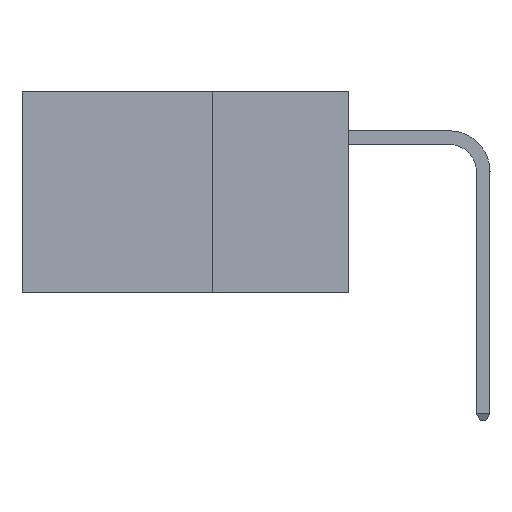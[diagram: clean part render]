
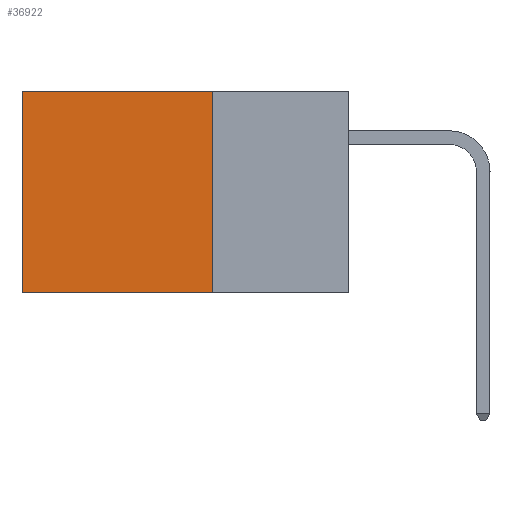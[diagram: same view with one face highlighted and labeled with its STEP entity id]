
A CAD part, left-side view. The second image highlights one B-rep face of the part: STEP entity #36922.
In plain terms, the highlighted planar face has unit normal (-1, 0, 0).
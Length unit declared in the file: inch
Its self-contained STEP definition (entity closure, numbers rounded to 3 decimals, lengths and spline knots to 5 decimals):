
#1063 = EDGE_CURVE ( 'NONE', #35926, #1633, #13323, .T. ) ;
#1204 = ORIENTED_EDGE ( 'NONE', *, *, #19303, .T. ) ;
#1633 = VERTEX_POINT ( 'NONE', #18950 ) ;
#6082 = CARTESIAN_POINT ( 'NONE',  ( 0.2875, 0.6, 0. ) ) ;
#7101 = CARTESIAN_POINT ( 'NONE',  ( 0.2875, 0.25, 0. ) ) ;
#8261 = VECTOR ( 'NONE', #16001, 39.37008 ) ;
#8582 = VECTOR ( 'NONE', #35623, 39.37008 ) ;
#9334 = VECTOR ( 'NONE', #11914, 39.37008 ) ;
#10995 = VERTEX_POINT ( 'NONE', #20126 ) ;
#11022 = EDGE_LOOP ( 'NONE', ( #1204, #17226, #28484, #34559 ) ) ;
#11562 = PLANE ( 'NONE',  #20854 ) ;
#11914 = DIRECTION ( 'NONE',  ( 0., 0., -1. ) ) ;
#13067 = CARTESIAN_POINT ( 'NONE',  ( 0.2875, 0.25, -0.37 ) ) ;
#13323 = LINE ( 'NONE', #7101, #28228 ) ;
#14456 = CARTESIAN_POINT ( 'NONE',  ( 0.2875, 0.25, 0. ) ) ;
#15670 = CARTESIAN_POINT ( 'NONE',  ( 0.2875, 0.25, 0. ) ) ;
#16001 = DIRECTION ( 'NONE',  ( 0., 1., 0. ) ) ;
#16380 = LINE ( 'NONE', #6082, #8582 ) ;
#17143 = LINE ( 'NONE', #20540, #9334 ) ;
#17226 = ORIENTED_EDGE ( 'NONE', *, *, #29145, .F. ) ;
#17474 = DIRECTION ( 'NONE',  ( 1., 0., 0. ) ) ;
#18248 = DIRECTION ( 'NONE',  ( 0., 1., 0. ) ) ;
#18950 = CARTESIAN_POINT ( 'NONE',  ( 0.2875, 0.6, 0. ) ) ;
#19303 = EDGE_CURVE ( 'NONE', #1633, #28948, #16380, .T. ) ;
#20126 = CARTESIAN_POINT ( 'NONE',  ( 0.2875, 0.25, -0.37 ) ) ;
#20540 = CARTESIAN_POINT ( 'NONE',  ( 0.2875, 0.25, 0. ) ) ;
#20807 = FACE_OUTER_BOUND ( 'NONE', #11022, .T. ) ;
#20854 = AXIS2_PLACEMENT_3D ( 'NONE', #14456, #17474, #38064 ) ;
#21396 = EDGE_CURVE ( 'NONE', #35926, #10995, #17143, .T. ) ;
#24955 = LINE ( 'NONE', #13067, #8261 ) ;
#28228 = VECTOR ( 'NONE', #18248, 39.37008 ) ;
#28484 = ORIENTED_EDGE ( 'NONE', *, *, #21396, .F. ) ;
#28948 = VERTEX_POINT ( 'NONE', #38078 ) ;
#29145 = EDGE_CURVE ( 'NONE', #10995, #28948, #24955, .T. ) ;
#34559 = ORIENTED_EDGE ( 'NONE', *, *, #1063, .T. ) ;
#35623 = DIRECTION ( 'NONE',  ( 0., 0., -1. ) ) ;
#35926 = VERTEX_POINT ( 'NONE', #15670 ) ;
#36922 = ADVANCED_FACE ( 'NONE', ( #20807 ), #11562, .F. ) ;
#38064 = DIRECTION ( 'NONE',  ( 0., 0., -1. ) ) ;
#38078 = CARTESIAN_POINT ( 'NONE',  ( 0.2875, 0.6, -0.37 ) ) ;
